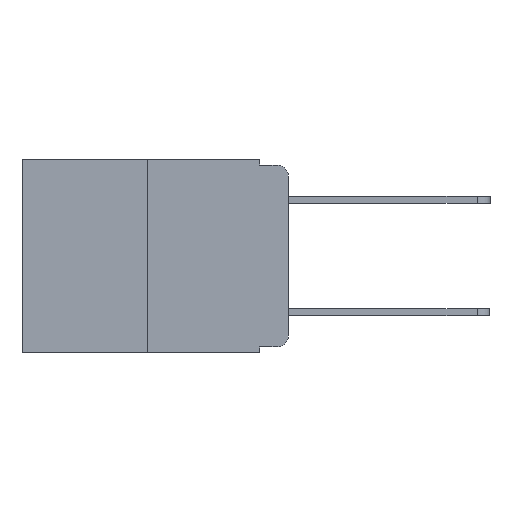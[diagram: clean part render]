
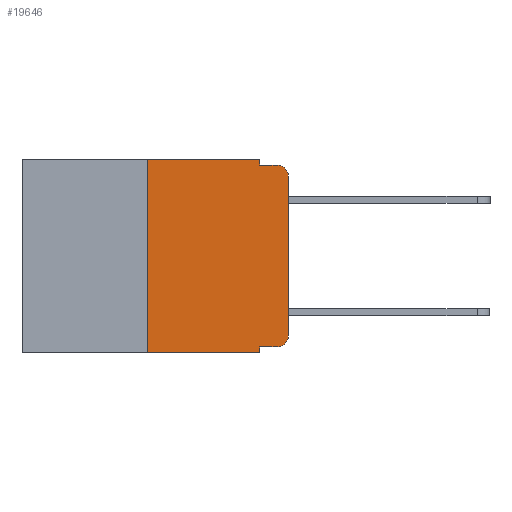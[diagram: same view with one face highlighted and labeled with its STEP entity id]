
A CAD part, left-side view. The second image highlights one B-rep face of the part: STEP entity #19646.
In plain terms, the highlighted planar face has unit normal (-1, 0, 0).
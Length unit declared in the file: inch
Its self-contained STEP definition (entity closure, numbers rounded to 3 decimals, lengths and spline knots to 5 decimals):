
#26 = DIRECTION ( 'NONE',  ( -1., 0., 0. ) ) ;
#40 = VECTOR ( 'NONE', #2737, 39.37008 ) ;
#183 = ORIENTED_EDGE ( 'NONE', *, *, #12887, .F. ) ;
#262 = VECTOR ( 'NONE', #6791, 39.37008 ) ;
#1002 = CARTESIAN_POINT ( 'NONE',  ( 0., 0.25, 0. ) ) ;
#1276 = ORIENTED_EDGE ( 'NONE', *, *, #2341, .F. ) ;
#1448 = EDGE_CURVE ( 'NONE', #19956, #7803, #14784, .T. ) ;
#1575 = CARTESIAN_POINT ( 'NONE',  ( 0., 0.051, -0.01 ) ) ;
#2060 = EDGE_CURVE ( 'NONE', #13163, #19205, #18007, .T. ) ;
#2067 = CARTESIAN_POINT ( 'NONE',  ( 0., 0.02, -0.313 ) ) ;
#2075 = AXIS2_PLACEMENT_3D ( 'NONE', #2067, #26, #22353 ) ;
#2120 = ORIENTED_EDGE ( 'NONE', *, *, #8166, .F. ) ;
#2154 = CARTESIAN_POINT ( 'NONE',  ( 0., 0.051, -0.343 ) ) ;
#2213 = PLANE ( 'NONE',  #9433 ) ;
#2341 = EDGE_CURVE ( 'NONE', #19205, #7148, #21212, .T. ) ;
#2417 = CARTESIAN_POINT ( 'NONE',  ( 0., 0.051, 0. ) ) ;
#2737 = DIRECTION ( 'NONE',  ( 0., 0., 1. ) ) ;
#3162 = VERTEX_POINT ( 'NONE', #20836 ) ;
#3979 = DIRECTION ( 'NONE',  ( 0., 0., -1. ) ) ;
#4265 = ORIENTED_EDGE ( 'NONE', *, *, #2060, .F. ) ;
#4508 = VERTEX_POINT ( 'NONE', #2154 ) ;
#4695 = EDGE_CURVE ( 'NONE', #20937, #13163, #9236, .T. ) ;
#4790 = CARTESIAN_POINT ( 'NONE',  ( 0., 0.02, -0.333 ) ) ;
#4808 = ORIENTED_EDGE ( 'NONE', *, *, #10458, .T. ) ;
#4886 = LINE ( 'NONE', #1575, #262 ) ;
#4910 = VECTOR ( 'NONE', #21277, 39.37008 ) ;
#5442 = ORIENTED_EDGE ( 'NONE', *, *, #4695, .F. ) ;
#5559 = LINE ( 'NONE', #6885, #9600 ) ;
#5613 = VECTOR ( 'NONE', #8112, 39.37008 ) ;
#6354 = CARTESIAN_POINT ( 'NONE',  ( 0., 0.051, 0. ) ) ;
#6791 = DIRECTION ( 'NONE',  ( 0., -1., 0. ) ) ;
#6885 = CARTESIAN_POINT ( 'NONE',  ( 0., 0.051, -0.333 ) ) ;
#7148 = VERTEX_POINT ( 'NONE', #17490 ) ;
#7475 = VECTOR ( 'NONE', #20496, 39.37008 ) ;
#7784 = DIRECTION ( 'NONE',  ( -1., 0., 0. ) ) ;
#7803 = VERTEX_POINT ( 'NONE', #20888 ) ;
#7825 = CARTESIAN_POINT ( 'NONE',  ( 0., 0., -0.03 ) ) ;
#8112 = DIRECTION ( 'NONE',  ( 0., 0., -1. ) ) ;
#8166 = EDGE_CURVE ( 'NONE', #16053, #4508, #13779, .T. ) ;
#8722 = ORIENTED_EDGE ( 'NONE', *, *, #20081, .T. ) ;
#9236 = LINE ( 'NONE', #1002, #40 ) ;
#9341 = CARTESIAN_POINT ( 'NONE',  ( 0., 0.25, -0.343 ) ) ;
#9433 = AXIS2_PLACEMENT_3D ( 'NONE', #21140, #14363, #3979 ) ;
#9439 = ORIENTED_EDGE ( 'NONE', *, *, #1448, .T. ) ;
#9600 = VECTOR ( 'NONE', #13832, 39.37008 ) ;
#10225 = ORIENTED_EDGE ( 'NONE', *, *, #12482, .T. ) ;
#10458 = EDGE_CURVE ( 'NONE', #14612, #3162, #13422, .T. ) ;
#10970 = CARTESIAN_POINT ( 'NONE',  ( 0., 0.473, -0.343 ) ) ;
#12407 = VECTOR ( 'NONE', #12552, 39.37008 ) ;
#12482 = EDGE_CURVE ( 'NONE', #20937, #4508, #13025, .T. ) ;
#12552 = DIRECTION ( 'NONE',  ( 0., 0., 1. ) ) ;
#12887 = EDGE_CURVE ( 'NONE', #7148, #3162, #4886, .T. ) ;
#13025 = LINE ( 'NONE', #10970, #4910 ) ;
#13163 = VERTEX_POINT ( 'NONE', #18103 ) ;
#13422 = CIRCLE ( 'NONE', #21986, 0.02 ) ;
#13482 = VECTOR ( 'NONE', #19770, 39.37008 ) ;
#13779 = LINE ( 'NONE', #6354, #5613 ) ;
#13832 = DIRECTION ( 'NONE',  ( 0., -1., 0. ) ) ;
#14363 = DIRECTION ( 'NONE',  ( 1., 0., 0. ) ) ;
#14612 = VERTEX_POINT ( 'NONE', #7825 ) ;
#14784 = CIRCLE ( 'NONE', #2075, 0.02 ) ;
#16053 = VERTEX_POINT ( 'NONE', #17220 ) ;
#17018 = LINE ( 'NONE', #19391, #12407 ) ;
#17077 = CARTESIAN_POINT ( 'NONE',  ( 0., 0.051, 0. ) ) ;
#17220 = CARTESIAN_POINT ( 'NONE',  ( 0., 0.051, -0.333 ) ) ;
#17490 = CARTESIAN_POINT ( 'NONE',  ( 0., 0.051, -0.01 ) ) ;
#17783 = EDGE_LOOP ( 'NONE', ( #19717, #4808, #183, #1276, #4265, #5442, #10225, #2120, #8722, #9439 ) ) ;
#17833 = EDGE_CURVE ( 'NONE', #7803, #14612, #17018, .T. ) ;
#18007 = LINE ( 'NONE', #20601, #13482 ) ;
#18095 = CARTESIAN_POINT ( 'NONE',  ( 0., 0.02, -0.03 ) ) ;
#18103 = CARTESIAN_POINT ( 'NONE',  ( 0., 0.25, 0. ) ) ;
#19205 = VERTEX_POINT ( 'NONE', #2417 ) ;
#19391 = CARTESIAN_POINT ( 'NONE',  ( 0., 0., 0. ) ) ;
#19646 = ADVANCED_FACE ( 'NONE', ( #21974 ), #2213, .F. ) ;
#19717 = ORIENTED_EDGE ( 'NONE', *, *, #17833, .T. ) ;
#19770 = DIRECTION ( 'NONE',  ( 0., -1., 0. ) ) ;
#19846 = DIRECTION ( 'NONE',  ( 0., 0., -1. ) ) ;
#19956 = VERTEX_POINT ( 'NONE', #4790 ) ;
#20081 = EDGE_CURVE ( 'NONE', #16053, #19956, #5559, .T. ) ;
#20496 = DIRECTION ( 'NONE',  ( 0., 0., -1. ) ) ;
#20601 = CARTESIAN_POINT ( 'NONE',  ( 0., 0.473, 0. ) ) ;
#20836 = CARTESIAN_POINT ( 'NONE',  ( 0., 0.02, -0.01 ) ) ;
#20888 = CARTESIAN_POINT ( 'NONE',  ( 0., 0., -0.313 ) ) ;
#20937 = VERTEX_POINT ( 'NONE', #9341 ) ;
#21140 = CARTESIAN_POINT ( 'NONE',  ( 0., 0.473, 0. ) ) ;
#21212 = LINE ( 'NONE', #17077, #7475 ) ;
#21277 = DIRECTION ( 'NONE',  ( 0., -1., 0. ) ) ;
#21974 = FACE_OUTER_BOUND ( 'NONE', #17783, .T. ) ;
#21986 = AXIS2_PLACEMENT_3D ( 'NONE', #18095, #7784, #19846 ) ;
#22353 = DIRECTION ( 'NONE',  ( 0., 0., -1. ) ) ;
